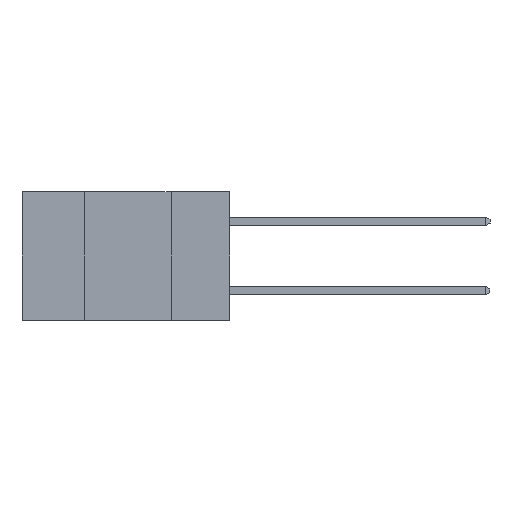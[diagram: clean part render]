
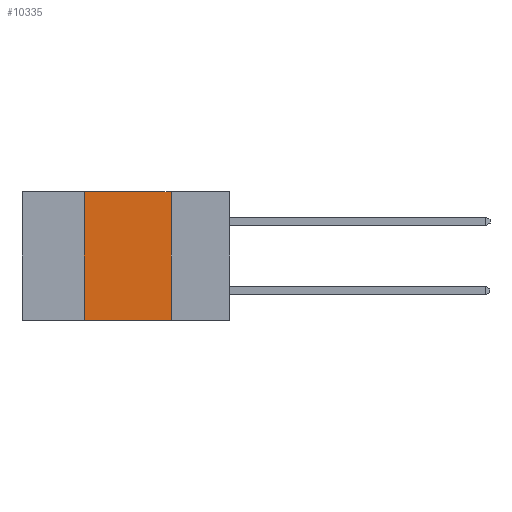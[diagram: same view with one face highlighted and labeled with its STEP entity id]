
A CAD part, left-side view. The second image highlights one B-rep face of the part: STEP entity #10335.
In plain terms, the highlighted planar face has unit normal (-1, 0, 0).
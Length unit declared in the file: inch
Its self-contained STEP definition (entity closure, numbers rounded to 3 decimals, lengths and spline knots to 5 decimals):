
#844 = CARTESIAN_POINT ( 'NONE',  ( 0., 0.17, -0.37 ) ) ;
#1008 = LINE ( 'NONE', #13857, #6807 ) ;
#1261 = DIRECTION ( 'NONE',  ( 0., 0., -1. ) ) ;
#1314 = EDGE_CURVE ( 'NONE', #8852, #10804, #1008, .T. ) ;
#1505 = CARTESIAN_POINT ( 'NONE',  ( 0., 0.42, 0. ) ) ;
#1948 = CARTESIAN_POINT ( 'NONE',  ( 0., 0.6, -0.37 ) ) ;
#3652 = DIRECTION ( 'NONE',  ( 0., -1., 0. ) ) ;
#4582 = DIRECTION ( 'NONE',  ( 1., 0., 0. ) ) ;
#4840 = AXIS2_PLACEMENT_3D ( 'NONE', #11039, #4582, #12093 ) ;
#5342 = LINE ( 'NONE', #1948, #7883 ) ;
#5641 = PLANE ( 'NONE',  #4840 ) ;
#5740 = EDGE_CURVE ( 'NONE', #8231, #10808, #11670, .T. ) ;
#6301 = VECTOR ( 'NONE', #9087, 39.37008 ) ;
#6807 = VECTOR ( 'NONE', #1261, 39.37008 ) ;
#7883 = VECTOR ( 'NONE', #9535, 39.37008 ) ;
#8004 = ORIENTED_EDGE ( 'NONE', *, *, #1314, .F. ) ;
#8231 = VERTEX_POINT ( 'NONE', #11221 ) ;
#8264 = ORIENTED_EDGE ( 'NONE', *, *, #13309, .F. ) ;
#8322 = ORIENTED_EDGE ( 'NONE', *, *, #5740, .F. ) ;
#8627 = ORIENTED_EDGE ( 'NONE', *, *, #10062, .T. ) ;
#8696 = EDGE_LOOP ( 'NONE', ( #8004, #8264, #8322, #8627 ) ) ;
#8852 = VERTEX_POINT ( 'NONE', #11020 ) ;
#9087 = DIRECTION ( 'NONE',  ( 0., 0., 1. ) ) ;
#9349 = VECTOR ( 'NONE', #3652, 39.37008 ) ;
#9513 = CARTESIAN_POINT ( 'NONE',  ( 0., 0.42, 0. ) ) ;
#9535 = DIRECTION ( 'NONE',  ( 0., -1., 0. ) ) ;
#9706 = LINE ( 'NONE', #12290, #9349 ) ;
#10062 = EDGE_CURVE ( 'NONE', #8231, #10804, #5342, .T. ) ;
#10335 = ADVANCED_FACE ( 'NONE', ( #12714 ), #5641, .F. ) ;
#10804 = VERTEX_POINT ( 'NONE', #844 ) ;
#10808 = VERTEX_POINT ( 'NONE', #9513 ) ;
#11020 = CARTESIAN_POINT ( 'NONE',  ( 0., 0.17, 0. ) ) ;
#11039 = CARTESIAN_POINT ( 'NONE',  ( 0., 0.6, 0. ) ) ;
#11221 = CARTESIAN_POINT ( 'NONE',  ( 0., 0.42, -0.37 ) ) ;
#11670 = LINE ( 'NONE', #1505, #6301 ) ;
#12093 = DIRECTION ( 'NONE',  ( 0., 0., -1. ) ) ;
#12290 = CARTESIAN_POINT ( 'NONE',  ( 0., 0.6, 0. ) ) ;
#12714 = FACE_OUTER_BOUND ( 'NONE', #8696, .T. ) ;
#13309 = EDGE_CURVE ( 'NONE', #10808, #8852, #9706, .T. ) ;
#13857 = CARTESIAN_POINT ( 'NONE',  ( 0., 0.17, 0. ) ) ;
